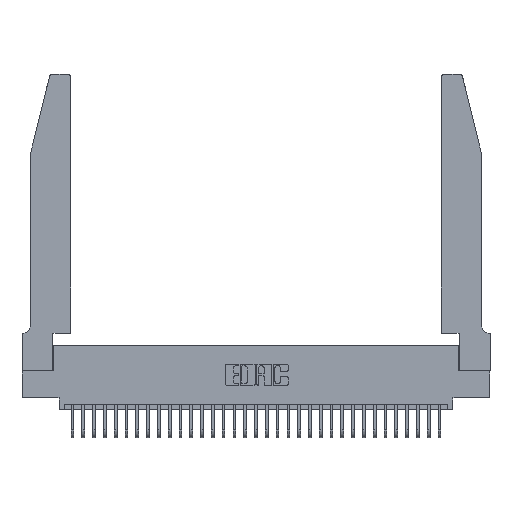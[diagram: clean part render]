
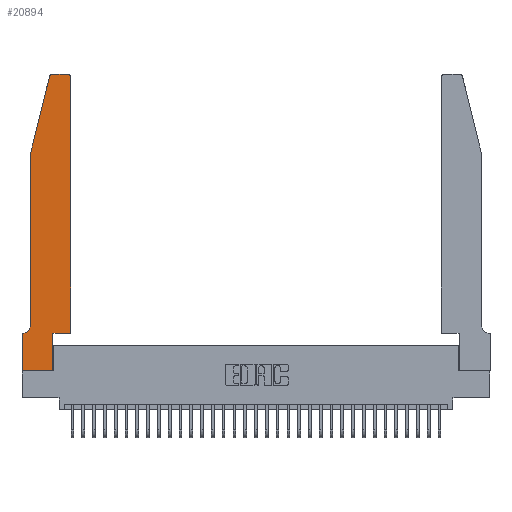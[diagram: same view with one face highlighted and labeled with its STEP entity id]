
A CAD part, top view. The second image highlights one B-rep face of the part: STEP entity #20894.
In plain terms, the highlighted planar face has unit normal (0, 0, 1).
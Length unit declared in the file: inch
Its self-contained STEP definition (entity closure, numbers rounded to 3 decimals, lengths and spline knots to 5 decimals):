
#778 = DIRECTION ( 'NONE',  ( 0., 0., 1. ) ) ;
#1023 = EDGE_CURVE ( 'NONE', #9835, #1199, #16962, .T. ) ;
#1199 = VERTEX_POINT ( 'NONE', #9791 ) ;
#1665 = LINE ( 'NONE', #14161, #14051 ) ;
#1700 = VERTEX_POINT ( 'NONE', #31617 ) ;
#1845 = ORIENTED_EDGE ( 'NONE', *, *, #17543, .T. ) ;
#2052 = EDGE_CURVE ( 'NONE', #29352, #9597, #17258, .T. ) ;
#2641 = CARTESIAN_POINT ( 'NONE',  ( 0.0055, 0.42, 0.37 ) ) ;
#2780 = CARTESIAN_POINT ( 'NONE',  ( 0.284, 2.72, 0.37 ) ) ;
#3084 = EDGE_CURVE ( 'NONE', #10339, #9835, #1665, .T. ) ;
#4396 = CIRCLE ( 'NONE', #11567, 0.03 ) ;
#4552 = LINE ( 'NONE', #26418, #17785 ) ;
#4576 = CARTESIAN_POINT ( 'NONE',  ( 0.0755, 0.35, 0.37 ) ) ;
#4637 = CARTESIAN_POINT ( 'NONE',  ( 0., 0.35, 0.37 ) ) ;
#4979 = ORIENTED_EDGE ( 'NONE', *, *, #26466, .T. ) ;
#5115 = DIRECTION ( 'NONE',  ( -1., 0., 0. ) ) ;
#5215 = VERTEX_POINT ( 'NONE', #27619 ) ;
#5297 = DIRECTION ( 'NONE',  ( 1., 0., 0. ) ) ;
#5815 = CARTESIAN_POINT ( 'NONE',  ( 0., 0., 0.37 ) ) ;
#7410 = CARTESIAN_POINT ( 'NONE',  ( 0.0055, 0.35, 0.37 ) ) ;
#7677 = LINE ( 'NONE', #4576, #13459 ) ;
#7751 = VECTOR ( 'NONE', #9075, 39.37008 ) ;
#8178 = CARTESIAN_POINT ( 'NONE',  ( 0.2865, 0., 0.37 ) ) ;
#8863 = AXIS2_PLACEMENT_3D ( 'NONE', #2641, #20042, #5115 ) ;
#8945 = EDGE_CURVE ( 'NONE', #1700, #17175, #20993, .T. ) ;
#9075 = DIRECTION ( 'NONE',  ( -1., 0., 0. ) ) ;
#9597 = VERTEX_POINT ( 'NONE', #7410 ) ;
#9791 = CARTESIAN_POINT ( 'NONE',  ( 0.4505, 2.72, 0.37 ) ) ;
#9835 = VERTEX_POINT ( 'NONE', #20667 ) ;
#10339 = VERTEX_POINT ( 'NONE', #27584 ) ;
#11403 = DIRECTION ( 'NONE',  ( 0., -1., 0. ) ) ;
#11567 = AXIS2_PLACEMENT_3D ( 'NONE', #2780, #20200, #5297 ) ;
#11779 = VECTOR ( 'NONE', #15846, 39.37008 ) ;
#12028 = EDGE_LOOP ( 'NONE', ( #28269, #30728, #4979, #19170, #20295, #16197, #25060, #24377, #17981, #26779, #31290, #1845 ) ) ;
#12097 = PLANE ( 'NONE',  #13102 ) ;
#12680 = EDGE_CURVE ( 'NONE', #14572, #10339, #19899, .T. ) ;
#13102 = AXIS2_PLACEMENT_3D ( 'NONE', #4637, #14605, #32116 ) ;
#13232 = VECTOR ( 'NONE', #23242, 39.37008 ) ;
#13459 = VECTOR ( 'NONE', #21782, 39.37008 ) ;
#13469 = EDGE_CURVE ( 'NONE', #26290, #14572, #29644, .T. ) ;
#13579 = VECTOR ( 'NONE', #13929, 39.37008 ) ;
#13929 = DIRECTION ( 'NONE',  ( -0.239, -0.971, 0. ) ) ;
#14051 = VECTOR ( 'NONE', #16672, 39.37008 ) ;
#14161 = CARTESIAN_POINT ( 'NONE',  ( 0.4505, 0.35, 0.37 ) ) ;
#14502 = CARTESIAN_POINT ( 'NONE',  ( 0.0755, 0.42, 0.37 ) ) ;
#14572 = VERTEX_POINT ( 'NONE', #8178 ) ;
#14605 = DIRECTION ( 'NONE',  ( 0., 0., 1. ) ) ;
#14904 = EDGE_CURVE ( 'NONE', #9597, #26711, #7677, .T. ) ;
#15585 = CARTESIAN_POINT ( 'NONE',  ( 0.4205, 2.72, 0.37 ) ) ;
#15846 = DIRECTION ( 'NONE',  ( 0., -1., 0. ) ) ;
#16197 = ORIENTED_EDGE ( 'NONE', *, *, #14904, .T. ) ;
#16672 = DIRECTION ( 'NONE',  ( 1., 0., 0. ) ) ;
#16961 = CARTESIAN_POINT ( 'NONE',  ( 0.25487, 2.72718, 0.37 ) ) ;
#16962 = LINE ( 'NONE', #26665, #29509 ) ;
#17175 = VERTEX_POINT ( 'NONE', #28879 ) ;
#17258 = CIRCLE ( 'NONE', #8863, 0.07 ) ;
#17543 = EDGE_CURVE ( 'NONE', #1199, #1700, #29415, .T. ) ;
#17785 = VECTOR ( 'NONE', #11403, 39.37008 ) ;
#17981 = ORIENTED_EDGE ( 'NONE', *, *, #12680, .T. ) ;
#17990 = EDGE_CURVE ( 'NONE', #17175, #32197, #4396, .T. ) ;
#18150 = DIRECTION ( 'NONE',  ( 1., 0., 0. ) ) ;
#18296 = CARTESIAN_POINT ( 'NONE',  ( 0.2865, 0.35, 0.37 ) ) ;
#18801 = CARTESIAN_POINT ( 'NONE',  ( 0., 0., 0.37 ) ) ;
#19170 = ORIENTED_EDGE ( 'NONE', *, *, #24146, .T. ) ;
#19235 = LINE ( 'NONE', #30866, #11779 ) ;
#19899 = LINE ( 'NONE', #18296, #13232 ) ;
#20042 = DIRECTION ( 'NONE',  ( 0., 0., -1. ) ) ;
#20200 = DIRECTION ( 'NONE',  ( 0., 0., 1. ) ) ;
#20250 = LINE ( 'NONE', #31446, #13579 ) ;
#20295 = ORIENTED_EDGE ( 'NONE', *, *, #2052, .T. ) ;
#20667 = CARTESIAN_POINT ( 'NONE',  ( 0.4505, 0.35, 0.37 ) ) ;
#20894 = ADVANCED_FACE ( 'NONE', ( #22262 ), #12097, .T. ) ;
#20993 = LINE ( 'NONE', #26555, #7751 ) ;
#21782 = DIRECTION ( 'NONE',  ( -1., 0., 0. ) ) ;
#22262 = FACE_OUTER_BOUND ( 'NONE', #12028, .T. ) ;
#23242 = DIRECTION ( 'NONE',  ( 0., 1., 0. ) ) ;
#23947 = DIRECTION ( 'NONE',  ( 1., 0., 0. ) ) ;
#24146 = EDGE_CURVE ( 'NONE', #5215, #29352, #4552, .T. ) ;
#24377 = ORIENTED_EDGE ( 'NONE', *, *, #13469, .T. ) ;
#24569 = AXIS2_PLACEMENT_3D ( 'NONE', #15585, #778, #18150 ) ;
#25060 = ORIENTED_EDGE ( 'NONE', *, *, #31939, .T. ) ;
#25533 = CARTESIAN_POINT ( 'NONE',  ( 0., 0.35, 0.37 ) ) ;
#26290 = VERTEX_POINT ( 'NONE', #5815 ) ;
#26418 = CARTESIAN_POINT ( 'NONE',  ( 0.0755, 2., 0.37 ) ) ;
#26466 = EDGE_CURVE ( 'NONE', #32197, #5215, #20250, .T. ) ;
#26555 = CARTESIAN_POINT ( 'NONE',  ( 0.2605, 2.75, 0.37 ) ) ;
#26665 = CARTESIAN_POINT ( 'NONE',  ( 0.4505, 0.35, 0.37 ) ) ;
#26711 = VERTEX_POINT ( 'NONE', #25533 ) ;
#26779 = ORIENTED_EDGE ( 'NONE', *, *, #3084, .T. ) ;
#27584 = CARTESIAN_POINT ( 'NONE',  ( 0.2865, 0.35, 0.37 ) ) ;
#27619 = CARTESIAN_POINT ( 'NONE',  ( 0.0755, 2., 0.37 ) ) ;
#28269 = ORIENTED_EDGE ( 'NONE', *, *, #8945, .T. ) ;
#28873 = VECTOR ( 'NONE', #23947, 39.37008 ) ;
#28879 = CARTESIAN_POINT ( 'NONE',  ( 0.284, 2.75, 0.37 ) ) ;
#29352 = VERTEX_POINT ( 'NONE', #14502 ) ;
#29415 = CIRCLE ( 'NONE', #24569, 0.03 ) ;
#29509 = VECTOR ( 'NONE', #31660, 39.37008 ) ;
#29644 = LINE ( 'NONE', #18801, #28873 ) ;
#30728 = ORIENTED_EDGE ( 'NONE', *, *, #17990, .T. ) ;
#30866 = CARTESIAN_POINT ( 'NONE',  ( 0., 0., 0.37 ) ) ;
#31290 = ORIENTED_EDGE ( 'NONE', *, *, #1023, .T. ) ;
#31446 = CARTESIAN_POINT ( 'NONE',  ( 0.0755, 2., 0.37 ) ) ;
#31617 = CARTESIAN_POINT ( 'NONE',  ( 0.4205, 2.75, 0.37 ) ) ;
#31660 = DIRECTION ( 'NONE',  ( 0., 1., 0. ) ) ;
#31939 = EDGE_CURVE ( 'NONE', #26711, #26290, #19235, .T. ) ;
#32116 = DIRECTION ( 'NONE',  ( 1., 0., 0. ) ) ;
#32197 = VERTEX_POINT ( 'NONE', #16961 ) ;
